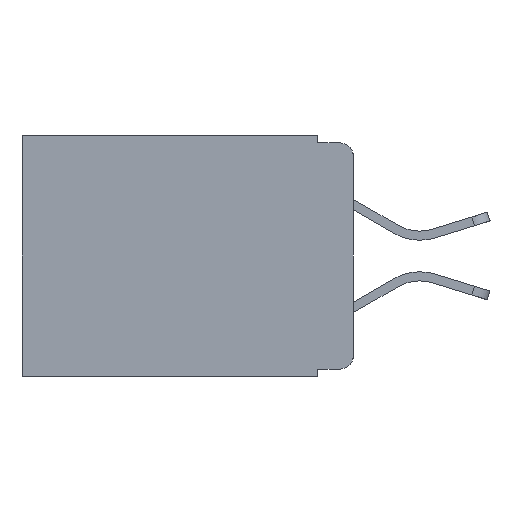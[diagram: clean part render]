
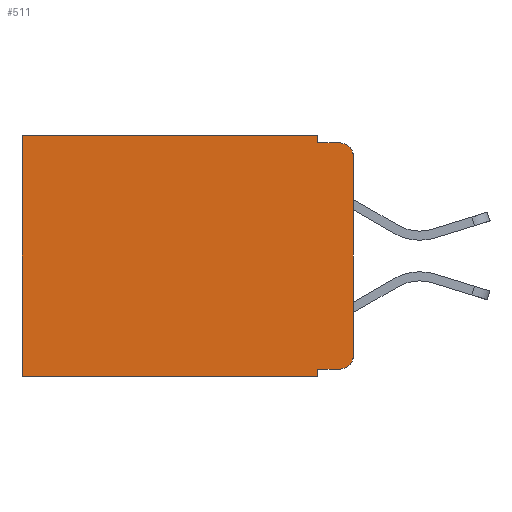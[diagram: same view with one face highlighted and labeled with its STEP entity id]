
A CAD part, left-side view. The second image highlights one B-rep face of the part: STEP entity #511.
In plain terms, the highlighted planar face has unit normal (-1, 0, 0).
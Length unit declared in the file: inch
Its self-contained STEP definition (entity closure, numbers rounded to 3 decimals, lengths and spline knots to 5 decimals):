
#48 = DIRECTION ( 'NONE',  ( 1., 0., 0. ) ) ;
#52 = VERTEX_POINT ( 'NONE', #10099 ) ;
#511 = ADVANCED_FACE ( 'NONE', ( #8573 ), #7938, .F. ) ;
#870 = DIRECTION ( 'NONE',  ( 0., 0., -1. ) ) ;
#928 = ORIENTED_EDGE ( 'NONE', *, *, #3243, .T. ) ;
#1128 = VERTEX_POINT ( 'NONE', #12027 ) ;
#1201 = VECTOR ( 'NONE', #8018, 39.37008 ) ;
#1221 = DIRECTION ( 'NONE',  ( 0., -1., 0. ) ) ;
#1591 = LINE ( 'NONE', #7199, #1201 ) ;
#1793 = VECTOR ( 'NONE', #5566, 39.37008 ) ;
#1844 = CARTESIAN_POINT ( 'NONE',  ( 0.298, 0.02, -0.333 ) ) ;
#2363 = DIRECTION ( 'NONE',  ( 0., 0., -1. ) ) ;
#2612 = CARTESIAN_POINT ( 'NONE',  ( 0.298, 0.473, 0. ) ) ;
#3137 = ORIENTED_EDGE ( 'NONE', *, *, #4051, .T. ) ;
#3198 = CARTESIAN_POINT ( 'NONE',  ( 0.298, 0.051, -0.343 ) ) ;
#3243 = EDGE_CURVE ( 'NONE', #1128, #3519, #3653, .T. ) ;
#3306 = ORIENTED_EDGE ( 'NONE', *, *, #4048, .F. ) ;
#3317 = AXIS2_PLACEMENT_3D ( 'NONE', #8930, #3440, #9727 ) ;
#3350 = VERTEX_POINT ( 'NONE', #3198 ) ;
#3440 = DIRECTION ( 'NONE',  ( -1., 0., 0. ) ) ;
#3519 = VERTEX_POINT ( 'NONE', #2612 ) ;
#3653 = LINE ( 'NONE', #5794, #8263 ) ;
#3817 = EDGE_CURVE ( 'NONE', #3350, #5974, #11554, .T. ) ;
#3883 = ORIENTED_EDGE ( 'NONE', *, *, #4010, .F. ) ;
#3965 = EDGE_CURVE ( 'NONE', #52, #5800, #1591, .T. ) ;
#3992 = EDGE_CURVE ( 'NONE', #52, #9864, #6491, .T. ) ;
#4010 = EDGE_CURVE ( 'NONE', #5885, #9864, #6196, .T. ) ;
#4013 = EDGE_CURVE ( 'NONE', #1128, #5885, #8229, .T. ) ;
#4032 = EDGE_CURVE ( 'NONE', #3519, #5974, #5656, .T. ) ;
#4048 = EDGE_CURVE ( 'NONE', #5427, #3350, #7707, .T. ) ;
#4050 = EDGE_CURVE ( 'NONE', #5427, #8585, #11812, .T. ) ;
#4051 = EDGE_CURVE ( 'NONE', #8585, #5800, #5057, .T. ) ;
#4316 = ORIENTED_EDGE ( 'NONE', *, *, #4050, .T. ) ;
#4591 = CARTESIAN_POINT ( 'NONE',  ( 0.298, 0., -0.343 ) ) ;
#4618 = CARTESIAN_POINT ( 'NONE',  ( 0.298, 0.051, 0. ) ) ;
#4704 = ORIENTED_EDGE ( 'NONE', *, *, #3817, .F. ) ;
#4765 = CARTESIAN_POINT ( 'NONE',  ( 0.298, 0., -0.313 ) ) ;
#5057 = CIRCLE ( 'NONE', #5389, 0.02 ) ;
#5389 = AXIS2_PLACEMENT_3D ( 'NONE', #10624, #5630, #11485 ) ;
#5427 = VERTEX_POINT ( 'NONE', #7134 ) ;
#5467 = CARTESIAN_POINT ( 'NONE',  ( 0.298, 0., 0. ) ) ;
#5502 = DIRECTION ( 'NONE',  ( 0., -1., 0. ) ) ;
#5548 = CARTESIAN_POINT ( 'NONE',  ( 0.298, 0.473, 0. ) ) ;
#5566 = DIRECTION ( 'NONE',  ( 0., 1., 0. ) ) ;
#5630 = DIRECTION ( 'NONE',  ( -1., 0., 0. ) ) ;
#5656 = LINE ( 'NONE', #5548, #9871 ) ;
#5794 = CARTESIAN_POINT ( 'NONE',  ( 0.298, 0., 0. ) ) ;
#5800 = VERTEX_POINT ( 'NONE', #4765 ) ;
#5802 = CARTESIAN_POINT ( 'NONE',  ( 0.298, 0.051, -0.01 ) ) ;
#5885 = VERTEX_POINT ( 'NONE', #5802 ) ;
#5924 = EDGE_LOOP ( 'NONE', ( #8876, #6880, #3883, #8685, #928, #9326, #4704, #3306, #4316, #3137 ) ) ;
#5933 = VECTOR ( 'NONE', #5502, 39.37008 ) ;
#5974 = VERTEX_POINT ( 'NONE', #10204 ) ;
#6196 = LINE ( 'NONE', #11374, #5933 ) ;
#6486 = CARTESIAN_POINT ( 'NONE',  ( 0.298, 0.051, -0.333 ) ) ;
#6491 = CIRCLE ( 'NONE', #3317, 0.02 ) ;
#6860 = DIRECTION ( 'NONE',  ( 0., 1., 0. ) ) ;
#6880 = ORIENTED_EDGE ( 'NONE', *, *, #3992, .T. ) ;
#7134 = CARTESIAN_POINT ( 'NONE',  ( 0.298, 0.051, -0.333 ) ) ;
#7199 = CARTESIAN_POINT ( 'NONE',  ( 0.298, 0., 0. ) ) ;
#7368 = DIRECTION ( 'NONE',  ( 0., 0., -1. ) ) ;
#7449 = VECTOR ( 'NONE', #7368, 39.37008 ) ;
#7707 = LINE ( 'NONE', #4618, #7449 ) ;
#7938 = PLANE ( 'NONE',  #8755 ) ;
#8018 = DIRECTION ( 'NONE',  ( 0., 0., -1. ) ) ;
#8098 = CARTESIAN_POINT ( 'NONE',  ( 0.298, 0.051, 0. ) ) ;
#8229 = LINE ( 'NONE', #8098, #12331 ) ;
#8263 = VECTOR ( 'NONE', #6860, 39.37008 ) ;
#8573 = FACE_OUTER_BOUND ( 'NONE', #5924, .T. ) ;
#8585 = VERTEX_POINT ( 'NONE', #1844 ) ;
#8685 = ORIENTED_EDGE ( 'NONE', *, *, #4013, .F. ) ;
#8755 = AXIS2_PLACEMENT_3D ( 'NONE', #5467, #48, #870 ) ;
#8876 = ORIENTED_EDGE ( 'NONE', *, *, #3965, .F. ) ;
#8930 = CARTESIAN_POINT ( 'NONE',  ( 0.298, 0.02, -0.03 ) ) ;
#9326 = ORIENTED_EDGE ( 'NONE', *, *, #4032, .T. ) ;
#9622 = VECTOR ( 'NONE', #1221, 39.37008 ) ;
#9727 = DIRECTION ( 'NONE',  ( 0., 0., -1. ) ) ;
#9864 = VERTEX_POINT ( 'NONE', #11860 ) ;
#9871 = VECTOR ( 'NONE', #12249, 39.37008 ) ;
#10099 = CARTESIAN_POINT ( 'NONE',  ( 0.298, 0., -0.03 ) ) ;
#10204 = CARTESIAN_POINT ( 'NONE',  ( 0.298, 0.473, -0.343 ) ) ;
#10624 = CARTESIAN_POINT ( 'NONE',  ( 0.298, 0.02, -0.313 ) ) ;
#11374 = CARTESIAN_POINT ( 'NONE',  ( 0.298, 0.051, -0.01 ) ) ;
#11485 = DIRECTION ( 'NONE',  ( 0., 0., -1. ) ) ;
#11554 = LINE ( 'NONE', #4591, #1793 ) ;
#11812 = LINE ( 'NONE', #6486, #9622 ) ;
#11860 = CARTESIAN_POINT ( 'NONE',  ( 0.298, 0.02, -0.01 ) ) ;
#12027 = CARTESIAN_POINT ( 'NONE',  ( 0.298, 0.051, 0. ) ) ;
#12249 = DIRECTION ( 'NONE',  ( 0., 0., -1. ) ) ;
#12331 = VECTOR ( 'NONE', #2363, 39.37008 ) ;
